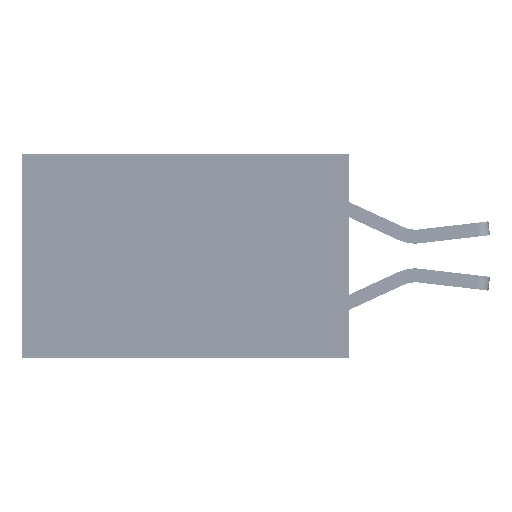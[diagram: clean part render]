
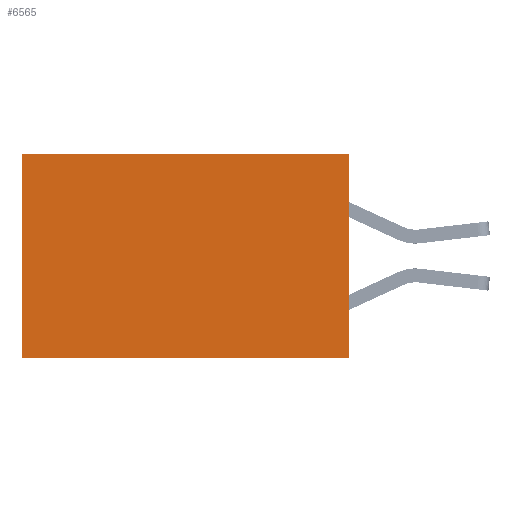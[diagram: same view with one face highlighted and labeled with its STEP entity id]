
A CAD part, left-side view. The second image highlights one B-rep face of the part: STEP entity #6565.
In plain terms, the highlighted planar face has unit normal (-1, 0, 0).
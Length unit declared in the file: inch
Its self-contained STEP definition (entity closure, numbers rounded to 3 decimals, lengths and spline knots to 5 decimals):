
#423 = FACE_OUTER_BOUND ( 'NONE', #27008, .T. ) ;
#552 = EDGE_CURVE ( 'NONE', #11942, #28730, #13152, .T. ) ;
#606 = DIRECTION ( 'NONE',  ( 0., 0., -1. ) ) ;
#1762 = VECTOR ( 'NONE', #29152, 39.37008 ) ;
#4608 = ORIENTED_EDGE ( 'NONE', *, *, #25249, .F. ) ;
#4657 = EDGE_CURVE ( 'NONE', #11942, #27525, #21370, .T. ) ;
#5095 = LINE ( 'NONE', #15362, #23544 ) ;
#5131 = AXIS2_PLACEMENT_3D ( 'NONE', #21239, #9056, #26119 ) ;
#6565 = ADVANCED_FACE ( 'NONE', ( #423 ), #6571, .F. ) ;
#6571 = PLANE ( 'NONE',  #5131 ) ;
#8810 = ORIENTED_EDGE ( 'NONE', *, *, #4657, .F. ) ;
#9056 = DIRECTION ( 'NONE',  ( 1., 0., 0. ) ) ;
#10982 = CARTESIAN_POINT ( 'NONE',  ( 0.277, 0., 0. ) ) ;
#11942 = VERTEX_POINT ( 'NONE', #10982 ) ;
#12614 = DIRECTION ( 'NONE',  ( 0., 1., 0. ) ) ;
#12976 = CARTESIAN_POINT ( 'NONE',  ( 0.277, 0., 0. ) ) ;
#13152 = LINE ( 'NONE', #12976, #25415 ) ;
#13760 = CARTESIAN_POINT ( 'NONE',  ( 0.277, 0., -0.37 ) ) ;
#13818 = CARTESIAN_POINT ( 'NONE',  ( 0.277, 0., -0.37 ) ) ;
#15362 = CARTESIAN_POINT ( 'NONE',  ( 0.277, 0.59, -0.37 ) ) ;
#15947 = ORIENTED_EDGE ( 'NONE', *, *, #24243, .T. ) ;
#18296 = ORIENTED_EDGE ( 'NONE', *, *, #552, .T. ) ;
#19070 = VERTEX_POINT ( 'NONE', #20458 ) ;
#20458 = CARTESIAN_POINT ( 'NONE',  ( 0.277, 0.59, -0.37 ) ) ;
#21171 = VECTOR ( 'NONE', #30754, 39.37008 ) ;
#21239 = CARTESIAN_POINT ( 'NONE',  ( 0.277, 0., -0.37 ) ) ;
#21370 = LINE ( 'NONE', #29188, #1762 ) ;
#23544 = VECTOR ( 'NONE', #606, 39.37008 ) ;
#24243 = EDGE_CURVE ( 'NONE', #28730, #19070, #5095, .T. ) ;
#25249 = EDGE_CURVE ( 'NONE', #27525, #19070, #27600, .T. ) ;
#25415 = VECTOR ( 'NONE', #12614, 39.37008 ) ;
#25880 = CARTESIAN_POINT ( 'NONE',  ( 0.277, 0.59, 0. ) ) ;
#26119 = DIRECTION ( 'NONE',  ( 0., 0., -1. ) ) ;
#27008 = EDGE_LOOP ( 'NONE', ( #15947, #4608, #8810, #18296 ) ) ;
#27525 = VERTEX_POINT ( 'NONE', #13760 ) ;
#27600 = LINE ( 'NONE', #13818, #21171 ) ;
#28730 = VERTEX_POINT ( 'NONE', #25880 ) ;
#29152 = DIRECTION ( 'NONE',  ( 0., 0., -1. ) ) ;
#29188 = CARTESIAN_POINT ( 'NONE',  ( 0.277, 0., -0.37 ) ) ;
#30754 = DIRECTION ( 'NONE',  ( 0., 1., 0. ) ) ;
